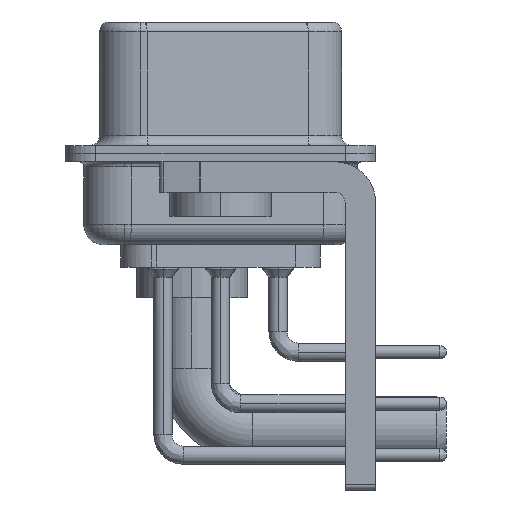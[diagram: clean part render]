
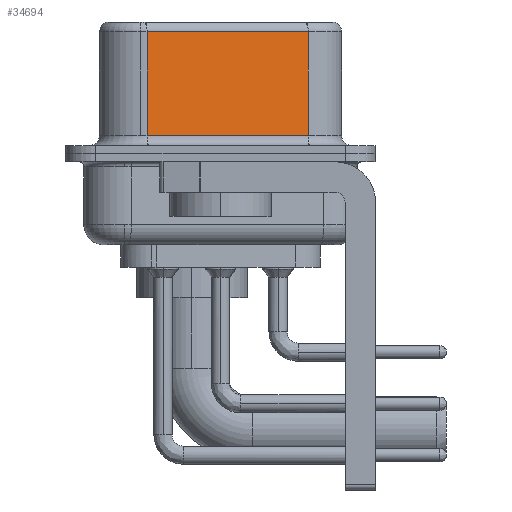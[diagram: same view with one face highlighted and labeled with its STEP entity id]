
A CAD part, left-side view. The second image highlights one B-rep face of the part: STEP entity #34694.
In plain terms, the highlighted planar face has unit normal (-0.985, -0.174, 0).
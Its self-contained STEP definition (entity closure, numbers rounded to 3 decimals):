
#870 = ORIENTED_EDGE ( 'NONE', *, *, #36979, .T. ) ;
#1288 = AXIS2_PLACEMENT_3D ( 'NONE', #24081, #32183, #12239 ) ;
#2887 = DIRECTION ( 'NONE',  ( 0.174, -0.985, 0. ) ) ;
#3109 = ORIENTED_EDGE ( 'NONE', *, *, #36057, .F. ) ;
#3273 = EDGE_CURVE ( 'NONE', #10740, #25453, #31502, .T. ) ;
#4337 = DIRECTION ( 'NONE',  ( -0.174, 0.985, 0. ) ) ;
#5232 = DIRECTION ( 'NONE',  ( 0., 0., -1. ) ) ;
#5276 = CARTESIAN_POINT ( 'NONE',  ( 5.132, -4.322, 6.02 ) ) ;
#5416 = CARTESIAN_POINT ( 'NONE',  ( 5.132, -4.322, 6.52 ) ) ;
#6699 = CARTESIAN_POINT ( 'NONE',  ( 5.132, -4.322, 0.9 ) ) ;
#7260 = VECTOR ( 'NONE', #5232, 1000. ) ;
#7534 = ORIENTED_EDGE ( 'NONE', *, *, #3273, .T. ) ;
#10740 = VERTEX_POINT ( 'NONE', #16433 ) ;
#12239 = DIRECTION ( 'NONE',  ( -0.174, 0.985, 0. ) ) ;
#15474 = VECTOR ( 'NONE', #35205, 1000. ) ;
#16433 = CARTESIAN_POINT ( 'NONE',  ( 3.73, 3.628, 0.9 ) ) ;
#16793 = EDGE_LOOP ( 'NONE', ( #3109, #870, #32110, #7534 ) ) ;
#17010 = VECTOR ( 'NONE', #2887, 1000. ) ;
#17866 = VERTEX_POINT ( 'NONE', #5276 ) ;
#18445 = LINE ( 'NONE', #33495, #30222 ) ;
#19536 = LINE ( 'NONE', #5416, #7260 ) ;
#20374 = CARTESIAN_POINT ( 'NONE',  ( 5.132, -4.322, 0.9 ) ) ;
#20875 = LINE ( 'NONE', #35760, #15474 ) ;
#24081 = CARTESIAN_POINT ( 'NONE',  ( 5.132, -4.322, 6.52 ) ) ;
#25453 = VERTEX_POINT ( 'NONE', #6699 ) ;
#26398 = VERTEX_POINT ( 'NONE', #32541 ) ;
#26542 = PLANE ( 'NONE',  #1288 ) ;
#29366 = FACE_OUTER_BOUND ( 'NONE', #16793, .T. ) ;
#30222 = VECTOR ( 'NONE', #4337, 1000. ) ;
#31232 = EDGE_CURVE ( 'NONE', #26398, #10740, #20875, .T. ) ;
#31502 = LINE ( 'NONE', #20374, #17010 ) ;
#32110 = ORIENTED_EDGE ( 'NONE', *, *, #31232, .T. ) ;
#32183 = DIRECTION ( 'NONE',  ( 0.985, 0.174, 0. ) ) ;
#32541 = CARTESIAN_POINT ( 'NONE',  ( 3.73, 3.628, 6.02 ) ) ;
#33495 = CARTESIAN_POINT ( 'NONE',  ( 5.132, -4.322, 6.02 ) ) ;
#34694 = ADVANCED_FACE ( 'NONE', ( #29366 ), #26542, .F. ) ;
#35205 = DIRECTION ( 'NONE',  ( 0., 0., -1. ) ) ;
#35760 = CARTESIAN_POINT ( 'NONE',  ( 3.73, 3.628, 6.52 ) ) ;
#36057 = EDGE_CURVE ( 'NONE', #17866, #25453, #19536, .T. ) ;
#36979 = EDGE_CURVE ( 'NONE', #17866, #26398, #18445, .T. ) ;
